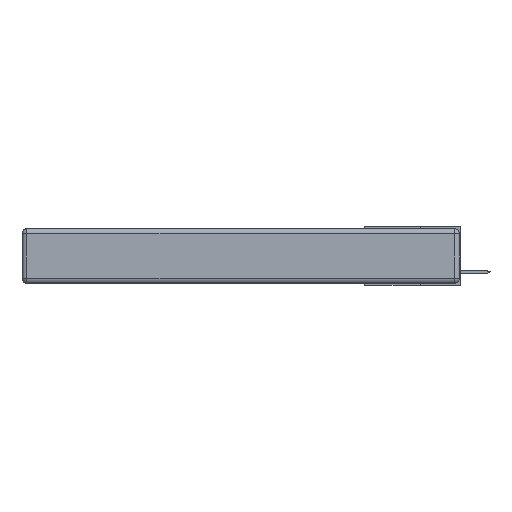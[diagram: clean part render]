
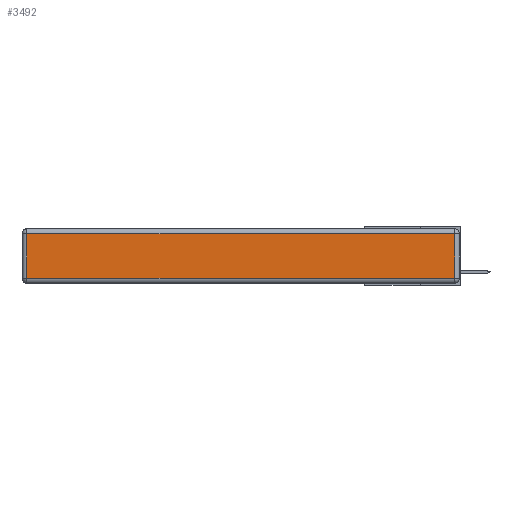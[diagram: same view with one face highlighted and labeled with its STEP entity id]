
A CAD part, left-side view. The second image highlights one B-rep face of the part: STEP entity #3492.
In plain terms, the highlighted planar face has unit normal (-1, 0, 0).
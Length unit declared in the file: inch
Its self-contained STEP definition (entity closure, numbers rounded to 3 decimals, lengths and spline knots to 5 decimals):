
#137 = PLANE ( 'NONE',  #10568 ) ;
#1184 = LINE ( 'NONE', #7209, #13727 ) ;
#1448 = DIRECTION ( 'NONE',  ( 0., 1., 0. ) ) ;
#2210 = LINE ( 'NONE', #18514, #19080 ) ;
#3492 = ADVANCED_FACE ( 'NONE', ( #3722 ), #137, .T. ) ;
#3722 = FACE_OUTER_BOUND ( 'NONE', #18327, .T. ) ;
#4653 = CARTESIAN_POINT ( 'NONE',  ( 0., 2.72, -0.313 ) ) ;
#5656 = EDGE_CURVE ( 'NONE', #17337, #14183, #11878, .T. ) ;
#6236 = EDGE_CURVE ( 'NONE', #7802, #17337, #2210, .T. ) ;
#6379 = DIRECTION ( 'NONE',  ( -1., 0., 0. ) ) ;
#7209 = CARTESIAN_POINT ( 'NONE',  ( 0., 0., -0.313 ) ) ;
#7802 = VERTEX_POINT ( 'NONE', #11388 ) ;
#7835 = EDGE_CURVE ( 'NONE', #14247, #7802, #1184, .T. ) ;
#9500 = CARTESIAN_POINT ( 'NONE',  ( 0., 0., -0.343 ) ) ;
#10568 = AXIS2_PLACEMENT_3D ( 'NONE', #9500, #6379, #13941 ) ;
#10683 = CARTESIAN_POINT ( 'NONE',  ( 0., 2.75, -0.03 ) ) ;
#11264 = LINE ( 'NONE', #12145, #13195 ) ;
#11388 = CARTESIAN_POINT ( 'NONE',  ( 0., 0.03, -0.313 ) ) ;
#11648 = CARTESIAN_POINT ( 'NONE',  ( 0., 2.72, -0.03 ) ) ;
#11878 = LINE ( 'NONE', #10683, #18140 ) ;
#12145 = CARTESIAN_POINT ( 'NONE',  ( 0., 2.72, -0.343 ) ) ;
#13195 = VECTOR ( 'NONE', #18476, 39.37008 ) ;
#13576 = EDGE_CURVE ( 'NONE', #14183, #14247, #11264, .T. ) ;
#13727 = VECTOR ( 'NONE', #19819, 39.37008 ) ;
#13823 = ORIENTED_EDGE ( 'NONE', *, *, #5656, .T. ) ;
#13941 = DIRECTION ( 'NONE',  ( 0., 0., 1. ) ) ;
#14183 = VERTEX_POINT ( 'NONE', #11648 ) ;
#14247 = VERTEX_POINT ( 'NONE', #4653 ) ;
#15812 = CARTESIAN_POINT ( 'NONE',  ( 0., 0.03, -0.03 ) ) ;
#17302 = ORIENTED_EDGE ( 'NONE', *, *, #7835, .T. ) ;
#17337 = VERTEX_POINT ( 'NONE', #15812 ) ;
#18140 = VECTOR ( 'NONE', #1448, 39.37008 ) ;
#18327 = EDGE_LOOP ( 'NONE', ( #17302, #18740, #13823, #19531 ) ) ;
#18476 = DIRECTION ( 'NONE',  ( 0., 0., -1. ) ) ;
#18514 = CARTESIAN_POINT ( 'NONE',  ( 0., 0.03, -0.343 ) ) ;
#18740 = ORIENTED_EDGE ( 'NONE', *, *, #6236, .T. ) ;
#19080 = VECTOR ( 'NONE', #19884, 39.37008 ) ;
#19531 = ORIENTED_EDGE ( 'NONE', *, *, #13576, .T. ) ;
#19819 = DIRECTION ( 'NONE',  ( 0., -1., 0. ) ) ;
#19884 = DIRECTION ( 'NONE',  ( 0., 0., 1. ) ) ;
